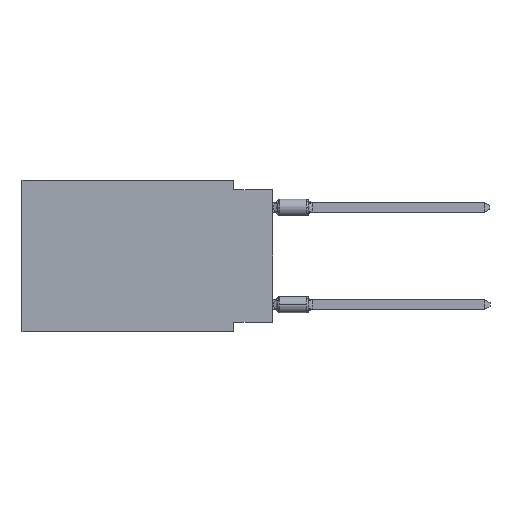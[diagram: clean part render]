
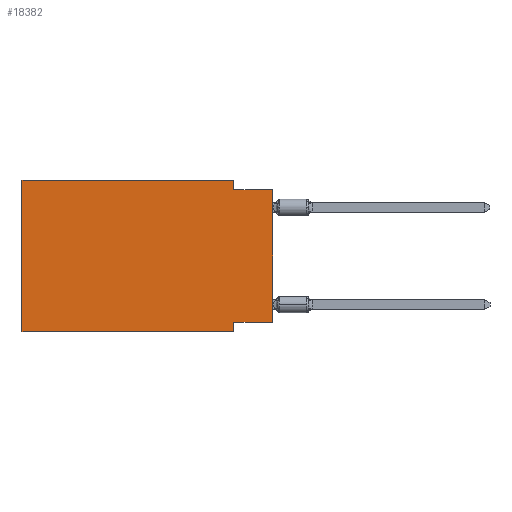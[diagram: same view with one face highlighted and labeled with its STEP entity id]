
A CAD part, left-side view. The second image highlights one B-rep face of the part: STEP entity #18382.
In plain terms, the highlighted planar face has unit normal (-1, 0, 0).
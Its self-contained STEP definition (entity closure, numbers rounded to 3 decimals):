
#45 = CARTESIAN_POINT ( 'NONE',  ( 0., 0., -9.271 ) ) ;
#419 = CARTESIAN_POINT ( 'NONE',  ( 0., 2.54, -9.271 ) ) ;
#421 = ORIENTED_EDGE ( 'NONE', *, *, #16700, .F. ) ;
#1133 = VERTEX_POINT ( 'NONE', #45 ) ;
#1301 = EDGE_LOOP ( 'NONE', ( #17706, #2537, #12538, #1755, #421, #15808, #18742, #8494 ) ) ;
#1313 = AXIS2_PLACEMENT_3D ( 'NONE', #16086, #6770, #16187 ) ;
#1755 = ORIENTED_EDGE ( 'NONE', *, *, #8091, .F. ) ;
#1963 = VERTEX_POINT ( 'NONE', #7924 ) ;
#2040 = CARTESIAN_POINT ( 'NONE',  ( 0., 2.54, -9.906 ) ) ;
#2537 = ORIENTED_EDGE ( 'NONE', *, *, #10844, .F. ) ;
#3363 = VECTOR ( 'NONE', #8538, 1000. ) ;
#3496 = DIRECTION ( 'NONE',  ( 0., -1., 0. ) ) ;
#3633 = EDGE_CURVE ( 'NONE', #14602, #7617, #16440, .T. ) ;
#4227 = DIRECTION ( 'NONE',  ( 0., 0., -1. ) ) ;
#4374 = DIRECTION ( 'NONE',  ( 0., -1., 0. ) ) ;
#4767 = VECTOR ( 'NONE', #15920, 1000. ) ;
#5005 = LINE ( 'NONE', #11165, #6491 ) ;
#5086 = CARTESIAN_POINT ( 'NONE',  ( 0., 0., 0. ) ) ;
#5655 = LINE ( 'NONE', #10102, #16103 ) ;
#5848 = VERTEX_POINT ( 'NONE', #419 ) ;
#6491 = VECTOR ( 'NONE', #3496, 1000. ) ;
#6770 = DIRECTION ( 'NONE',  ( 1., 0., 0. ) ) ;
#6850 = VECTOR ( 'NONE', #9312, 1000. ) ;
#6951 = VERTEX_POINT ( 'NONE', #9285 ) ;
#7617 = VERTEX_POINT ( 'NONE', #13397 ) ;
#7824 = VECTOR ( 'NONE', #4227, 1000. ) ;
#7924 = CARTESIAN_POINT ( 'NONE',  ( 0., 0., -0.635 ) ) ;
#8091 = EDGE_CURVE ( 'NONE', #6951, #18310, #15195, .T. ) ;
#8494 = ORIENTED_EDGE ( 'NONE', *, *, #19965, .F. ) ;
#8538 = DIRECTION ( 'NONE',  ( 0., -1., 0. ) ) ;
#8881 = DIRECTION ( 'NONE',  ( 0., 0., 1. ) ) ;
#9285 = CARTESIAN_POINT ( 'NONE',  ( 0., 16.383, 0. ) ) ;
#9312 = DIRECTION ( 'NONE',  ( 0., 0., 1. ) ) ;
#10102 = CARTESIAN_POINT ( 'NONE',  ( 0., 16.383, 0. ) ) ;
#10378 = CARTESIAN_POINT ( 'NONE',  ( 0., 16.383, -9.906 ) ) ;
#10447 = EDGE_CURVE ( 'NONE', #18310, #14377, #10890, .T. ) ;
#10844 = EDGE_CURVE ( 'NONE', #14377, #1963, #5005, .T. ) ;
#10890 = LINE ( 'NONE', #12812, #13263 ) ;
#11165 = CARTESIAN_POINT ( 'NONE',  ( 0., 0., -0.635 ) ) ;
#11199 = CARTESIAN_POINT ( 'NONE',  ( 0., 2.54, -0.635 ) ) ;
#11633 = FACE_OUTER_BOUND ( 'NONE', #1301, .T. ) ;
#11920 = VECTOR ( 'NONE', #4374, 1000. ) ;
#12344 = EDGE_CURVE ( 'NONE', #1133, #1963, #14180, .T. ) ;
#12538 = ORIENTED_EDGE ( 'NONE', *, *, #10447, .F. ) ;
#12812 = CARTESIAN_POINT ( 'NONE',  ( 0., 2.54, 0. ) ) ;
#12907 = EDGE_CURVE ( 'NONE', #5848, #7617, #14946, .T. ) ;
#13263 = VECTOR ( 'NONE', #18971, 1000. ) ;
#13397 = CARTESIAN_POINT ( 'NONE',  ( 0., 2.54, -9.906 ) ) ;
#13514 = PLANE ( 'NONE',  #1313 ) ;
#14180 = LINE ( 'NONE', #5086, #6850 ) ;
#14377 = VERTEX_POINT ( 'NONE', #11199 ) ;
#14602 = VERTEX_POINT ( 'NONE', #10378 ) ;
#14623 = CARTESIAN_POINT ( 'NONE',  ( 0., 16.383, -9.906 ) ) ;
#14671 = CARTESIAN_POINT ( 'NONE',  ( 0., 2.54, 0. ) ) ;
#14946 = LINE ( 'NONE', #2040, #7824 ) ;
#15195 = LINE ( 'NONE', #16809, #11920 ) ;
#15808 = ORIENTED_EDGE ( 'NONE', *, *, #3633, .T. ) ;
#15920 = DIRECTION ( 'NONE',  ( 0., 1., 0. ) ) ;
#16086 = CARTESIAN_POINT ( 'NONE',  ( 0., 16.383, 0. ) ) ;
#16103 = VECTOR ( 'NONE', #8881, 1000. ) ;
#16187 = DIRECTION ( 'NONE',  ( 0., 0., -1. ) ) ;
#16440 = LINE ( 'NONE', #14623, #3363 ) ;
#16700 = EDGE_CURVE ( 'NONE', #14602, #6951, #5655, .T. ) ;
#16809 = CARTESIAN_POINT ( 'NONE',  ( 0., 16.383, 0. ) ) ;
#17129 = CARTESIAN_POINT ( 'NONE',  ( 0., 0., -9.271 ) ) ;
#17522 = LINE ( 'NONE', #17129, #4767 ) ;
#17706 = ORIENTED_EDGE ( 'NONE', *, *, #12344, .T. ) ;
#18310 = VERTEX_POINT ( 'NONE', #14671 ) ;
#18382 = ADVANCED_FACE ( 'NONE', ( #11633 ), #13514, .F. ) ;
#18742 = ORIENTED_EDGE ( 'NONE', *, *, #12907, .F. ) ;
#18971 = DIRECTION ( 'NONE',  ( 0., 0., -1. ) ) ;
#19965 = EDGE_CURVE ( 'NONE', #1133, #5848, #17522, .T. ) ;
